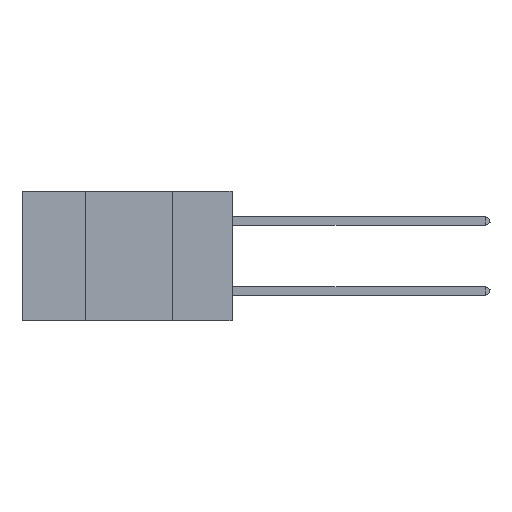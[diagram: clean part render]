
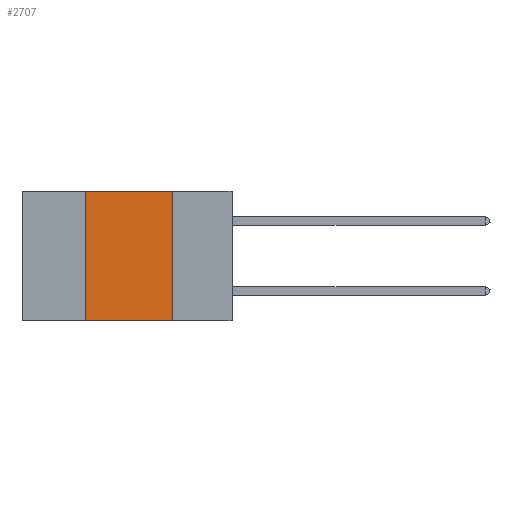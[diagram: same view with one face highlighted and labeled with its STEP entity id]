
A CAD part, left-side view. The second image highlights one B-rep face of the part: STEP entity #2707.
In plain terms, the highlighted planar face has unit normal (-1, 0, 0).
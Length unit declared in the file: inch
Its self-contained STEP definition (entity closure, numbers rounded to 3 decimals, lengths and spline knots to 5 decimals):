
#775 = ORIENTED_EDGE ( 'NONE', *, *, #14030, .F. ) ;
#2578 = VECTOR ( 'NONE', #14537, 39.37008 ) ;
#2707 = ADVANCED_FACE ( 'NONE', ( #6242 ), #22691, .F. ) ;
#3861 = CARTESIAN_POINT ( 'NONE',  ( 0., 0.6, -0.37 ) ) ;
#4031 = ORIENTED_EDGE ( 'NONE', *, *, #32417, .T. ) ;
#4260 = VECTOR ( 'NONE', #32711, 39.37008 ) ;
#5848 = EDGE_CURVE ( 'NONE', #16625, #25009, #11188, .T. ) ;
#6242 = FACE_OUTER_BOUND ( 'NONE', #25523, .T. ) ;
#7454 = CARTESIAN_POINT ( 'NONE',  ( 0., 0.42, 0. ) ) ;
#9347 = ORIENTED_EDGE ( 'NONE', *, *, #10960, .F. ) ;
#9770 = DIRECTION ( 'NONE',  ( 1., 0., 0. ) ) ;
#10960 = EDGE_CURVE ( 'NONE', #18045, #18351, #21417, .T. ) ;
#11188 = LINE ( 'NONE', #17253, #4260 ) ;
#11360 = DIRECTION ( 'NONE',  ( 0., -1., 0. ) ) ;
#13405 = CARTESIAN_POINT ( 'NONE',  ( 0., 0.17, -0.37 ) ) ;
#13907 = CARTESIAN_POINT ( 'NONE',  ( 0., 0.42, 0. ) ) ;
#14030 = EDGE_CURVE ( 'NONE', #18351, #16625, #27044, .T. ) ;
#14537 = DIRECTION ( 'NONE',  ( 0., -1., 0. ) ) ;
#16625 = VERTEX_POINT ( 'NONE', #26453 ) ;
#16660 = CARTESIAN_POINT ( 'NONE',  ( 0., 0.42, -0.37 ) ) ;
#17253 = CARTESIAN_POINT ( 'NONE',  ( 0., 0.17, 0. ) ) ;
#18045 = VERTEX_POINT ( 'NONE', #16660 ) ;
#18351 = VERTEX_POINT ( 'NONE', #7454 ) ;
#21417 = LINE ( 'NONE', #13907, #33395 ) ;
#22691 = PLANE ( 'NONE',  #31666 ) ;
#24088 = LINE ( 'NONE', #3861, #2578 ) ;
#24248 = CARTESIAN_POINT ( 'NONE',  ( 0., 0.6, 0. ) ) ;
#25009 = VERTEX_POINT ( 'NONE', #13405 ) ;
#25253 = CARTESIAN_POINT ( 'NONE',  ( 0., 0.6, 0. ) ) ;
#25523 = EDGE_LOOP ( 'NONE', ( #27538, #775, #9347, #4031 ) ) ;
#26453 = CARTESIAN_POINT ( 'NONE',  ( 0., 0.17, 0. ) ) ;
#27044 = LINE ( 'NONE', #24248, #32213 ) ;
#27538 = ORIENTED_EDGE ( 'NONE', *, *, #5848, .F. ) ;
#27841 = DIRECTION ( 'NONE',  ( 0., 0., -1. ) ) ;
#31666 = AXIS2_PLACEMENT_3D ( 'NONE', #25253, #9770, #27841 ) ;
#31928 = DIRECTION ( 'NONE',  ( 0., 0., 1. ) ) ;
#32213 = VECTOR ( 'NONE', #11360, 39.37008 ) ;
#32417 = EDGE_CURVE ( 'NONE', #18045, #25009, #24088, .T. ) ;
#32711 = DIRECTION ( 'NONE',  ( 0., 0., -1. ) ) ;
#33395 = VECTOR ( 'NONE', #31928, 39.37008 ) ;
